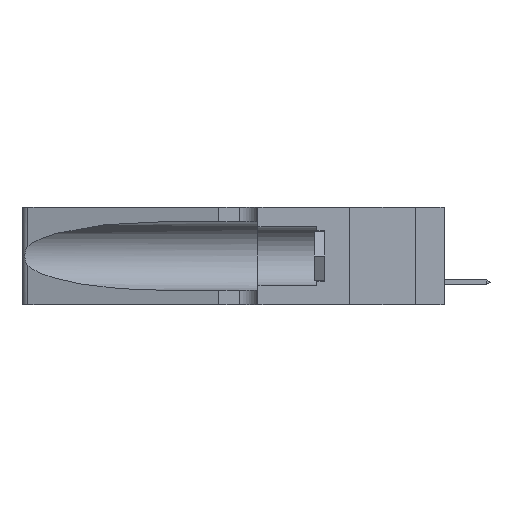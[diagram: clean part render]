
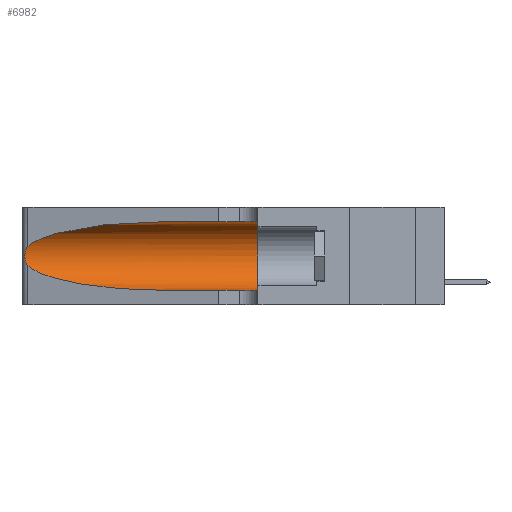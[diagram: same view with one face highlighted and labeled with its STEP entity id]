
A CAD part, left-side view. The second image highlights one B-rep face of the part: STEP entity #6982.
In plain terms, the highlighted cylindrical face has radius 3.308 mm (diameter 6.617 mm), a partial arc.
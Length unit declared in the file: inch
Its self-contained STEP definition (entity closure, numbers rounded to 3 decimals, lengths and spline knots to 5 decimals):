
#222 = CARTESIAN_POINT ( 'NONE',  ( 0.25487, 1.22718, 0.14631 ) ) ;
#363 = VERTEX_POINT ( 'NONE', #5598 ) ;
#497 = CARTESIAN_POINT ( 'NONE',  ( 0.18966, 0.96281, 0.31525 ) ) ;
#914 = ORIENTED_EDGE ( 'NONE', *, *, #8820, .T. ) ;
#2077 = DIRECTION ( 'NONE',  ( 0., -1., 0. ) ) ;
#2636 = CARTESIAN_POINT ( 'NONE',  ( 0.2373, 1.15595, 0.28018 ) ) ;
#2835 = B_SPLINE_CURVE_WITH_KNOTS ( 'NONE', 3,
 ( #7678, #22875, #26900, #7767, #24903, #20523, #11907, #24993, #18528, #9745, #11998, #25082, #5525, #14276 ),
 .UNSPECIFIED., .F., .F.,
 ( 4, 2, 2, 2, 2, 2, 4 ),
 ( 0., 0.00027, 0.00053, 0.00107, 0.0016, 0.00187, 0.00214 ),
 .UNSPECIFIED. ) ;
#2909 = FACE_OUTER_BOUND ( 'NONE', #3859, .T. ) ;
#3503 = DIRECTION ( 'NONE',  ( 0., 0., -1. ) ) ;
#3859 = EDGE_LOOP ( 'NONE', ( #10375, #25095, #914, #21994, #7657, #26261 ) ) ;
#4608 = CIRCLE ( 'NONE', #12820, 0.13025 ) ;
#4657 = LINE ( 'NONE', #14877, #9357 ) ;
#5204 = DIRECTION ( 'NONE',  ( 0., -1., 0. ) ) ;
#5525 = CARTESIAN_POINT ( 'NONE',  ( 0.25555, 1.22993, 0.14849 ) ) ;
#5598 = CARTESIAN_POINT ( 'NONE',  ( 0.1305, 0.35, 0.05475 ) ) ;
#6982 = ADVANCED_FACE ( 'NONE', ( #2909 ), #10294, .F. ) ;
#7057 = CARTESIAN_POINT ( 'NONE',  ( 0.2373, 1.15595, 0.08982 ) ) ;
#7148 = AXIS2_PLACEMENT_3D ( 'NONE', #18111, #5204, #3503 ) ;
#7657 = ORIENTED_EDGE ( 'NONE', *, *, #12864, .F. ) ;
#7678 = CARTESIAN_POINT ( 'NONE',  ( 0.25487, 1.22718, 0.22369 ) ) ;
#7767 = CARTESIAN_POINT ( 'NONE',  ( 0.25787, 1.23484, 0.2124 ) ) ;
#8820 = EDGE_CURVE ( 'NONE', #18451, #20140, #14927, .T. ) ;
#9357 = VECTOR ( 'NONE', #21019, 39.37008 ) ;
#9745 = CARTESIAN_POINT ( 'NONE',  ( 0.25856, 1.23593, 0.16098 ) ) ;
#9905 = CARTESIAN_POINT ( 'NONE',  ( 0.1305, 0.35, 0.185 ) ) ;
#10196 = DIRECTION ( 'NONE',  ( 0., 0., 1. ) ) ;
#10294 = CYLINDRICAL_SURFACE ( 'NONE', #7148, 0.13025 ) ;
#10375 = ORIENTED_EDGE ( 'NONE', *, *, #17115, .T. ) ;
#10917 = CARTESIAN_POINT ( 'NONE',  ( 0.18966, 0.96281, 0.05475 ) ) ;
#11434 = VERTEX_POINT ( 'NONE', #17629 ) ;
#11907 = CARTESIAN_POINT ( 'NONE',  ( 0.26075, 1.23896, 0.19203 ) ) ;
#11998 = CARTESIAN_POINT ( 'NONE',  ( 0.25789, 1.23486, 0.15765 ) ) ;
#12064 = EDGE_CURVE ( 'NONE', #20140, #363, #4657, .T. ) ;
#12338 = CARTESIAN_POINT ( 'NONE',  ( 0.1305, 0.72297, 0.05475 ) ) ;
#12820 = AXIS2_PLACEMENT_3D ( 'NONE', #9905, #20968, #10196 ) ;
#12864 = EDGE_CURVE ( 'NONE', #27625, #363, #4608, .T. ) ;
#13072 = CARTESIAN_POINT ( 'NONE',  ( 0.1305, 0.72297, 0.05475 ) ) ;
#14276 = CARTESIAN_POINT ( 'NONE',  ( 0.25487, 1.22718, 0.14631 ) ) ;
#14877 = CARTESIAN_POINT ( 'NONE',  ( 0.1305, 1.61858, 0.05475 ) ) ;
#14927 =( BOUNDED_CURVE ( )  B_SPLINE_CURVE ( 3, ( #222, #7057, #10917, #13072 ),
 .UNSPECIFIED., .F., .F. ) 
 B_SPLINE_CURVE_WITH_KNOTS ( ( 4, 4 ),
 ( 3.44316, 4.71239 ),
 .UNSPECIFIED. ) 
 CURVE ( )  GEOMETRIC_REPRESENTATION_ITEM ( )  RATIONAL_B_SPLINE_CURVE ( ( 1., 0.87, 0.87, 1. ) ) 
 REPRESENTATION_ITEM ( '' )  );
#17039 = EDGE_CURVE ( 'NONE', #11434, #27625, #23327, .T. ) ;
#17115 = EDGE_CURVE ( 'NONE', #11434, #24848, #21168, .T. ) ;
#17629 = CARTESIAN_POINT ( 'NONE',  ( 0.1305, 0.72297, 0.31525 ) ) ;
#18111 = CARTESIAN_POINT ( 'NONE',  ( 0.1305, 1.61858, 0.185 ) ) ;
#18451 = VERTEX_POINT ( 'NONE', #24022 ) ;
#18528 = CARTESIAN_POINT ( 'NONE',  ( 0.26017, 1.23833, 0.17102 ) ) ;
#19704 = CARTESIAN_POINT ( 'NONE',  ( 0.25487, 1.22718, 0.22369 ) ) ;
#20140 = VERTEX_POINT ( 'NONE', #12338 ) ;
#20523 = CARTESIAN_POINT ( 'NONE',  ( 0.26018, 1.23835, 0.19895 ) ) ;
#20740 = CARTESIAN_POINT ( 'NONE',  ( 0.25487, 1.22718, 0.22369 ) ) ;
#20968 = DIRECTION ( 'NONE',  ( 0., 1., 0. ) ) ;
#21019 = DIRECTION ( 'NONE',  ( 0., -1., 0. ) ) ;
#21108 = CARTESIAN_POINT ( 'NONE',  ( 0.1305, 0.35, 0.31525 ) ) ;
#21168 =( BOUNDED_CURVE ( )  B_SPLINE_CURVE ( 3, ( #26179, #497, #2636, #19704 ),
 .UNSPECIFIED., .F., .F. ) 
 B_SPLINE_CURVE_WITH_KNOTS ( ( 4, 4 ),
 ( 1.5708, 2.84003 ),
 .UNSPECIFIED. ) 
 CURVE ( )  GEOMETRIC_REPRESENTATION_ITEM ( )  RATIONAL_B_SPLINE_CURVE ( ( 1., 0.87, 0.87, 1. ) ) 
 REPRESENTATION_ITEM ( '' )  );
#21994 = ORIENTED_EDGE ( 'NONE', *, *, #12064, .T. ) ;
#22875 = CARTESIAN_POINT ( 'NONE',  ( 0.25555, 1.22994, 0.2215 ) ) ;
#23327 = LINE ( 'NONE', #27769, #24335 ) ;
#24022 = CARTESIAN_POINT ( 'NONE',  ( 0.25487, 1.22718, 0.14631 ) ) ;
#24335 = VECTOR ( 'NONE', #2077, 39.37008 ) ;
#24848 = VERTEX_POINT ( 'NONE', #20740 ) ;
#24903 = CARTESIAN_POINT ( 'NONE',  ( 0.25854, 1.2359, 0.20912 ) ) ;
#24993 = CARTESIAN_POINT ( 'NONE',  ( 0.26075, 1.23896, 0.178 ) ) ;
#25082 = CARTESIAN_POINT ( 'NONE',  ( 0.25639, 1.23186, 0.15144 ) ) ;
#25095 = ORIENTED_EDGE ( 'NONE', *, *, #25321, .T. ) ;
#25321 = EDGE_CURVE ( 'NONE', #24848, #18451, #2835, .T. ) ;
#26179 = CARTESIAN_POINT ( 'NONE',  ( 0.1305, 0.72297, 0.31525 ) ) ;
#26261 = ORIENTED_EDGE ( 'NONE', *, *, #17039, .F. ) ;
#26900 = CARTESIAN_POINT ( 'NONE',  ( 0.25639, 1.23184, 0.21858 ) ) ;
#27625 = VERTEX_POINT ( 'NONE', #21108 ) ;
#27769 = CARTESIAN_POINT ( 'NONE',  ( 0.1305, 1.61858, 0.31525 ) ) ;
